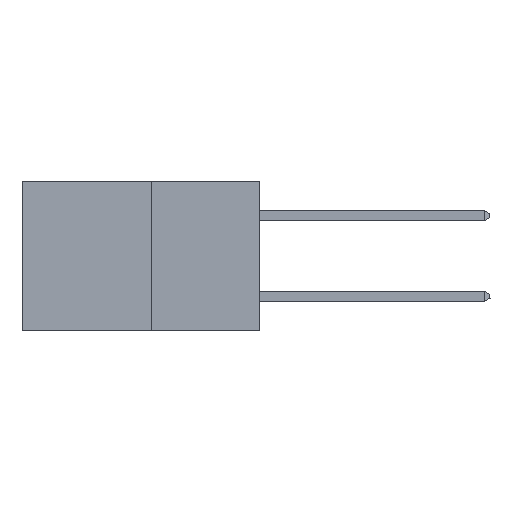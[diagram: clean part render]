
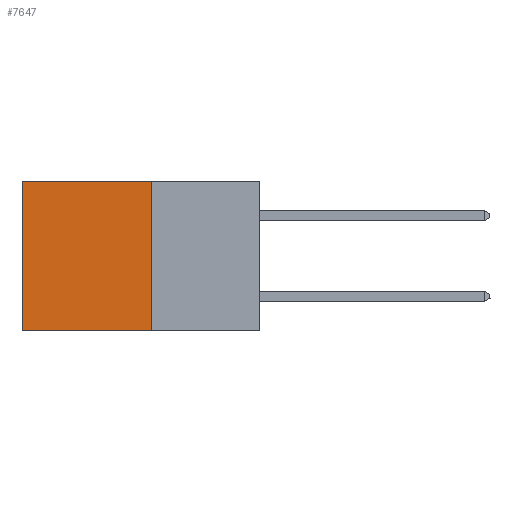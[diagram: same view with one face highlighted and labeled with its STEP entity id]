
A CAD part, left-side view. The second image highlights one B-rep face of the part: STEP entity #7647.
In plain terms, the highlighted planar face has unit normal (-1, 0, 0).
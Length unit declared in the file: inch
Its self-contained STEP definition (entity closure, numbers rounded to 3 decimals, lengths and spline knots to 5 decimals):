
#2352 = LINE ( 'NONE', #6919, #22694 ) ;
#2609 = DIRECTION ( 'NONE',  ( 0., 0., -1. ) ) ;
#3255 = CARTESIAN_POINT ( 'NONE',  ( 0.277, 0.59, -0.37 ) ) ;
#3312 = CARTESIAN_POINT ( 'NONE',  ( 0.277, 0.27, -0.37 ) ) ;
#4039 = VERTEX_POINT ( 'NONE', #3312 ) ;
#4640 = VERTEX_POINT ( 'NONE', #3255 ) ;
#4971 = AXIS2_PLACEMENT_3D ( 'NONE', #22393, #17241, #22457 ) ;
#5146 = EDGE_LOOP ( 'NONE', ( #10825, #19515, #5887, #9171 ) ) ;
#5189 = CARTESIAN_POINT ( 'NONE',  ( 0.277, 0.59, 0. ) ) ;
#5887 = ORIENTED_EDGE ( 'NONE', *, *, #9198, .F. ) ;
#6919 = CARTESIAN_POINT ( 'NONE',  ( 0.277, 0.27, -0.37 ) ) ;
#7642 = DIRECTION ( 'NONE',  ( 0., 1., 0. ) ) ;
#7647 = ADVANCED_FACE ( 'NONE', ( #11206 ), #22095, .F. ) ;
#7759 = CARTESIAN_POINT ( 'NONE',  ( 0.277, 0.59, -0.37 ) ) ;
#7824 = VECTOR ( 'NONE', #7642, 39.37008 ) ;
#9127 = LINE ( 'NONE', #21670, #7824 ) ;
#9151 = VERTEX_POINT ( 'NONE', #26227 ) ;
#9171 = ORIENTED_EDGE ( 'NONE', *, *, #21997, .T. ) ;
#9198 = EDGE_CURVE ( 'NONE', #9151, #4039, #2352, .T. ) ;
#10825 = ORIENTED_EDGE ( 'NONE', *, *, #21309, .T. ) ;
#11206 = FACE_OUTER_BOUND ( 'NONE', #5146, .T. ) ;
#11565 = CARTESIAN_POINT ( 'NONE',  ( 0.277, 0.27, -0.37 ) ) ;
#12827 = VERTEX_POINT ( 'NONE', #5189 ) ;
#16019 = VECTOR ( 'NONE', #23590, 39.37008 ) ;
#17241 = DIRECTION ( 'NONE',  ( 1., 0., 0. ) ) ;
#18882 = VECTOR ( 'NONE', #21787, 39.37008 ) ;
#19515 = ORIENTED_EDGE ( 'NONE', *, *, #26223, .F. ) ;
#20668 = LINE ( 'NONE', #11565, #16019 ) ;
#21309 = EDGE_CURVE ( 'NONE', #12827, #4640, #23614, .T. ) ;
#21670 = CARTESIAN_POINT ( 'NONE',  ( 0.277, 0.27, 0. ) ) ;
#21787 = DIRECTION ( 'NONE',  ( 0., 0., -1. ) ) ;
#21997 = EDGE_CURVE ( 'NONE', #9151, #12827, #9127, .T. ) ;
#22095 = PLANE ( 'NONE',  #4971 ) ;
#22393 = CARTESIAN_POINT ( 'NONE',  ( 0.277, 0.27, -0.37 ) ) ;
#22457 = DIRECTION ( 'NONE',  ( 0., 0., -1. ) ) ;
#22694 = VECTOR ( 'NONE', #2609, 39.37008 ) ;
#23590 = DIRECTION ( 'NONE',  ( 0., 1., 0. ) ) ;
#23614 = LINE ( 'NONE', #7759, #18882 ) ;
#26223 = EDGE_CURVE ( 'NONE', #4039, #4640, #20668, .T. ) ;
#26227 = CARTESIAN_POINT ( 'NONE',  ( 0.277, 0.27, 0. ) ) ;
